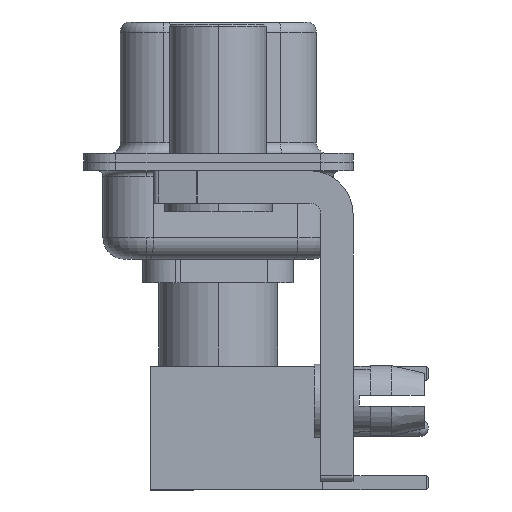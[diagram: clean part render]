
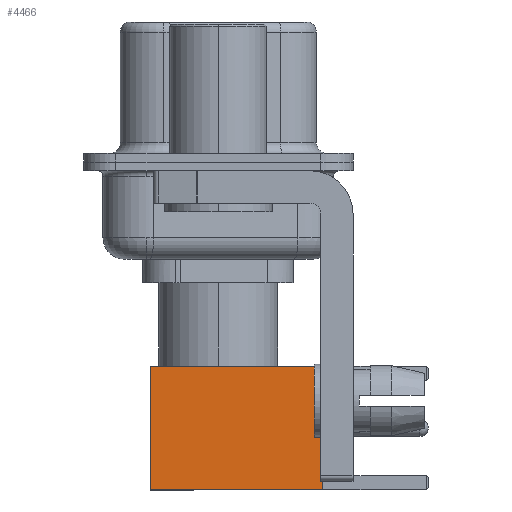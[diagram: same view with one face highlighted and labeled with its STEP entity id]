
A CAD part, left-side view. The second image highlights one B-rep face of the part: STEP entity #4466.
In plain terms, the highlighted face is planar.
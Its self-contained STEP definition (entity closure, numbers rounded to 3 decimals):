
#93 = LINE ( 'NONE', #6344, #19079 ) ;
#1070 = CARTESIAN_POINT ( 'NONE',  ( 2.875, 2.875, 0. ) ) ;
#2083 = CARTESIAN_POINT ( 'NONE',  ( 2.875, 2.875, 8. ) ) ;
#2408 = DIRECTION ( 'NONE',  ( 0., 0., 1. ) ) ;
#3578 = LINE ( 'NONE', #10237, #16760 ) ;
#4466 = ADVANCED_FACE ( 'NONE', ( #10671 ), #5897, .T. ) ;
#4860 = CARTESIAN_POINT ( 'NONE',  ( -2.875, 2.875, 8. ) ) ;
#5076 = DIRECTION ( 'NONE',  ( -1., 0., 0. ) ) ;
#5162 = EDGE_CURVE ( 'NONE', #13271, #20202, #93, .T. ) ;
#5897 = PLANE ( 'NONE',  #9859 ) ;
#6344 = CARTESIAN_POINT ( 'NONE',  ( 0., 2.875, 0. ) ) ;
#6425 = ORIENTED_EDGE ( 'NONE', *, *, #9950, .T. ) ;
#8205 = DIRECTION ( 'NONE',  ( -1., 0., 0. ) ) ;
#8875 = CARTESIAN_POINT ( 'NONE',  ( -2.875, 2.875, 0. ) ) ;
#9345 = DIRECTION ( 'NONE',  ( 0., 0., -1. ) ) ;
#9859 = AXIS2_PLACEMENT_3D ( 'NONE', #19083, #17183, #2408 ) ;
#9950 = EDGE_CURVE ( 'NONE', #15162, #13271, #14047, .T. ) ;
#10237 = CARTESIAN_POINT ( 'NONE',  ( 0., 2.875, 8. ) ) ;
#10671 = FACE_OUTER_BOUND ( 'NONE', #19069, .T. ) ;
#11860 = DIRECTION ( 'NONE',  ( 0., 0., -1. ) ) ;
#12049 = VECTOR ( 'NONE', #9345, 1000. ) ;
#12242 = EDGE_CURVE ( 'NONE', #13541, #20202, #18688, .T. ) ;
#13271 = VERTEX_POINT ( 'NONE', #14035 ) ;
#13541 = VERTEX_POINT ( 'NONE', #4860 ) ;
#13757 = ORIENTED_EDGE ( 'NONE', *, *, #5162, .T. ) ;
#14035 = CARTESIAN_POINT ( 'NONE',  ( 2.875, 2.875, 0. ) ) ;
#14047 = LINE ( 'NONE', #1070, #12049 ) ;
#15162 = VERTEX_POINT ( 'NONE', #2083 ) ;
#15232 = EDGE_CURVE ( 'NONE', #15162, #13541, #3578, .T. ) ;
#16760 = VECTOR ( 'NONE', #8205, 1000. ) ;
#16769 = VECTOR ( 'NONE', #11860, 1000. ) ;
#17183 = DIRECTION ( 'NONE',  ( 0., 1., 0. ) ) ;
#17630 = ORIENTED_EDGE ( 'NONE', *, *, #12242, .F. ) ;
#18688 = LINE ( 'NONE', #8875, #16769 ) ;
#18842 = ORIENTED_EDGE ( 'NONE', *, *, #15232, .F. ) ;
#19069 = EDGE_LOOP ( 'NONE', ( #6425, #13757, #17630, #18842 ) ) ;
#19079 = VECTOR ( 'NONE', #5076, 1000. ) ;
#19083 = CARTESIAN_POINT ( 'NONE',  ( 2.875, 2.875, 0. ) ) ;
#20202 = VERTEX_POINT ( 'NONE', #20742 ) ;
#20742 = CARTESIAN_POINT ( 'NONE',  ( -2.875, 2.875, 0. ) ) ;
